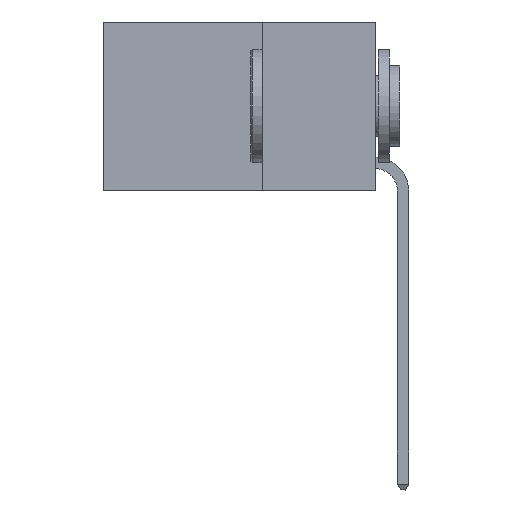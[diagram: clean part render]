
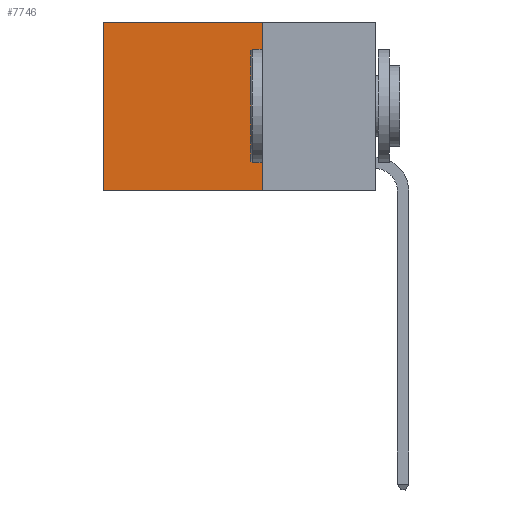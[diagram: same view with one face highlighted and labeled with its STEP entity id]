
A CAD part, left-side view. The second image highlights one B-rep face of the part: STEP entity #7746.
In plain terms, the highlighted planar face has unit normal (-1, 0, 0).
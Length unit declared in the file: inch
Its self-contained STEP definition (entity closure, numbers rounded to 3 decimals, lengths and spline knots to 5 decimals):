
#52 = VERTEX_POINT ( 'NONE', #4726 ) ;
#209 = ORIENTED_EDGE ( 'NONE', *, *, #5595, .F. ) ;
#442 = AXIS2_PLACEMENT_3D ( 'NONE', #15717, #17043, #9027 ) ;
#791 = ORIENTED_EDGE ( 'NONE', *, *, #10255, .T. ) ;
#3690 = VERTEX_POINT ( 'NONE', #4124 ) ;
#4124 = CARTESIAN_POINT ( 'NONE',  ( 0.2625, 0.6, 0. ) ) ;
#4726 = CARTESIAN_POINT ( 'NONE',  ( 0.2625, 0.25, 0. ) ) ;
#5595 = EDGE_CURVE ( 'NONE', #16416, #6128, #16697, .T. ) ;
#5627 = VECTOR ( 'NONE', #9092, 39.37008 ) ;
#5845 = DIRECTION ( 'NONE',  ( 0., 0., -1. ) ) ;
#6008 = CARTESIAN_POINT ( 'NONE',  ( 0.2625, 0.25, -0.37 ) ) ;
#6128 = VERTEX_POINT ( 'NONE', #12431 ) ;
#6276 = PLANE ( 'NONE',  #442 ) ;
#6336 = CARTESIAN_POINT ( 'NONE',  ( 0.2625, 0.25, 0. ) ) ;
#7262 = CARTESIAN_POINT ( 'NONE',  ( 0.2625, 0.25, -0.37 ) ) ;
#7746 = ADVANCED_FACE ( 'NONE', ( #17233 ), #6276, .F. ) ;
#7768 = EDGE_CURVE ( 'NONE', #52, #16416, #9283, .T. ) ;
#8723 = CARTESIAN_POINT ( 'NONE',  ( 0.2625, 0.25, 0. ) ) ;
#9027 = DIRECTION ( 'NONE',  ( 0., 0., -1. ) ) ;
#9092 = DIRECTION ( 'NONE',  ( 0., 0., -1. ) ) ;
#9210 = EDGE_LOOP ( 'NONE', ( #791, #209, #11458, #11158 ) ) ;
#9283 = LINE ( 'NONE', #6336, #5627 ) ;
#9811 = VECTOR ( 'NONE', #5845, 39.37008 ) ;
#10255 = EDGE_CURVE ( 'NONE', #3690, #6128, #15701, .T. ) ;
#11158 = ORIENTED_EDGE ( 'NONE', *, *, #15817, .T. ) ;
#11458 = ORIENTED_EDGE ( 'NONE', *, *, #7768, .F. ) ;
#12431 = CARTESIAN_POINT ( 'NONE',  ( 0.2625, 0.6, -0.37 ) ) ;
#13141 = VECTOR ( 'NONE', #16657, 39.37008 ) ;
#13143 = VECTOR ( 'NONE', #15421, 39.37008 ) ;
#13578 = LINE ( 'NONE', #8723, #13143 ) ;
#13981 = CARTESIAN_POINT ( 'NONE',  ( 0.2625, 0.6, 0. ) ) ;
#15421 = DIRECTION ( 'NONE',  ( 0., 1., 0. ) ) ;
#15701 = LINE ( 'NONE', #13981, #9811 ) ;
#15717 = CARTESIAN_POINT ( 'NONE',  ( 0.2625, 0.25, 0. ) ) ;
#15817 = EDGE_CURVE ( 'NONE', #52, #3690, #13578, .T. ) ;
#16416 = VERTEX_POINT ( 'NONE', #6008 ) ;
#16657 = DIRECTION ( 'NONE',  ( 0., 1., 0. ) ) ;
#16697 = LINE ( 'NONE', #7262, #13141 ) ;
#17043 = DIRECTION ( 'NONE',  ( 1., 0., 0. ) ) ;
#17233 = FACE_OUTER_BOUND ( 'NONE', #9210, .T. ) ;
